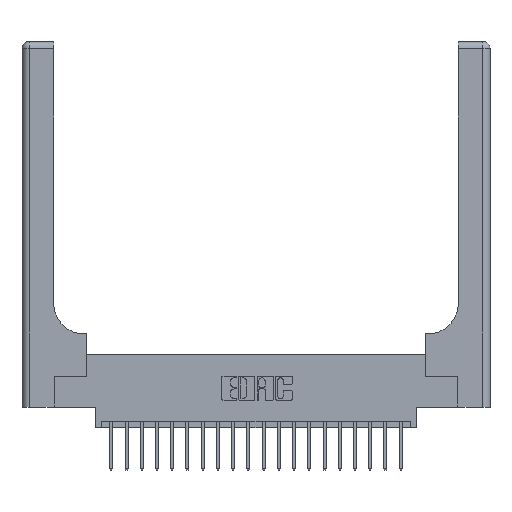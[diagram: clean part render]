
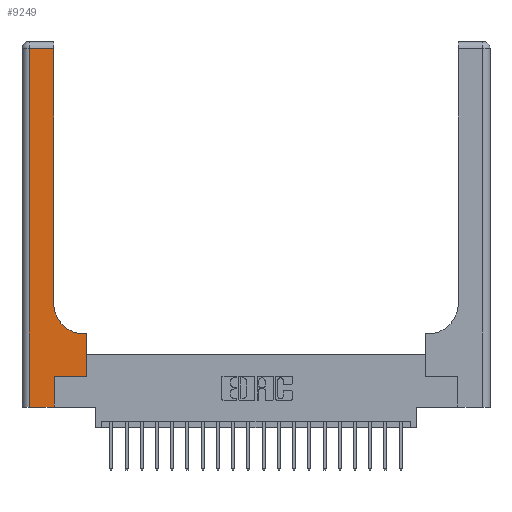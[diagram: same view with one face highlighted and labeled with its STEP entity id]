
A CAD part, top view. The second image highlights one B-rep face of the part: STEP entity #9249.
In plain terms, the highlighted planar face has unit normal (0, 0, 1).
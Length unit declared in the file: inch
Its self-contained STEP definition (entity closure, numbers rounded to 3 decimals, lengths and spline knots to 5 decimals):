
#969 = ORIENTED_EDGE ( 'NONE', *, *, #4519, .T. ) ;
#1064 = CARTESIAN_POINT ( 'NONE',  ( 0.51, 0.6, 0.37 ) ) ;
#1404 = PLANE ( 'NONE',  #8314 ) ;
#1443 = VECTOR ( 'NONE', #10503, 39.37008 ) ;
#1856 = ORIENTED_EDGE ( 'NONE', *, *, #5648, .T. ) ;
#2175 = CARTESIAN_POINT ( 'NONE',  ( 0.26, 3., 0.37 ) ) ;
#2435 = CARTESIAN_POINT ( 'NONE',  ( 0.26, 0.85, 0.37 ) ) ;
#2613 = CARTESIAN_POINT ( 'NONE',  ( 0.26, 0.6, 0.37 ) ) ;
#3101 = DIRECTION ( 'NONE',  ( 0., 0., -1. ) ) ;
#3227 = DIRECTION ( 'NONE',  ( 0., 0., -1. ) ) ;
#3654 = VERTEX_POINT ( 'NONE', #8436 ) ;
#4396 = LINE ( 'NONE', #18512, #11097 ) ;
#4419 = VERTEX_POINT ( 'NONE', #5235 ) ;
#4519 = EDGE_CURVE ( 'NONE', #6497, #8329, #18994, .T. ) ;
#4797 = VECTOR ( 'NONE', #16852, 39.37008 ) ;
#5235 = CARTESIAN_POINT ( 'NONE',  ( 0.265, 0., 0.37 ) ) ;
#5289 = VERTEX_POINT ( 'NONE', #1064 ) ;
#5648 = EDGE_CURVE ( 'NONE', #20893, #11310, #8142, .T. ) ;
#5678 = CARTESIAN_POINT ( 'NONE',  ( 0.265, 0.25, 0.37 ) ) ;
#5838 = CARTESIAN_POINT ( 'NONE',  ( 0.528, 0.25, 0.37 ) ) ;
#6059 = LINE ( 'NONE', #2613, #14283 ) ;
#6120 = CARTESIAN_POINT ( 'NONE',  ( 0.528, 0.6, 0.37 ) ) ;
#6497 = VERTEX_POINT ( 'NONE', #2435 ) ;
#6508 = EDGE_LOOP ( 'NONE', ( #969, #9099, #1856, #19226, #16027, #8920, #12571, #19442, #12322 ) ) ;
#6956 = CARTESIAN_POINT ( 'NONE',  ( 0.265, 0., 0.37 ) ) ;
#7095 = DIRECTION ( 'NONE',  ( 1., 0., 0. ) ) ;
#7485 = DIRECTION ( 'NONE',  ( 0., 1., 0. ) ) ;
#7694 = EDGE_CURVE ( 'NONE', #13878, #5289, #6059, .T. ) ;
#7697 = EDGE_CURVE ( 'NONE', #8329, #20893, #19194, .T. ) ;
#7995 = CIRCLE ( 'NONE', #12030, 0.25 ) ;
#8142 = LINE ( 'NONE', #15171, #4797 ) ;
#8241 = EDGE_CURVE ( 'NONE', #11310, #4419, #9414, .T. ) ;
#8314 = AXIS2_PLACEMENT_3D ( 'NONE', #16167, #3101, #14602 ) ;
#8329 = VERTEX_POINT ( 'NONE', #8822 ) ;
#8365 = VECTOR ( 'NONE', #7095, 39.37008 ) ;
#8436 = CARTESIAN_POINT ( 'NONE',  ( 0.528, 0.25, 0.37 ) ) ;
#8703 = CARTESIAN_POINT ( 'NONE',  ( 0.06, 0., 0.37 ) ) ;
#8822 = CARTESIAN_POINT ( 'NONE',  ( 0.26, 2.94, 0.37 ) ) ;
#8920 = ORIENTED_EDGE ( 'NONE', *, *, #10804, .T. ) ;
#9099 = ORIENTED_EDGE ( 'NONE', *, *, #7697, .T. ) ;
#9249 = ADVANCED_FACE ( 'NONE', ( #20881 ), #1404, .F. ) ;
#9271 = DIRECTION ( 'NONE',  ( -1., 0., 0. ) ) ;
#9414 = LINE ( 'NONE', #18601, #8365 ) ;
#9637 = VERTEX_POINT ( 'NONE', #5678 ) ;
#10503 = DIRECTION ( 'NONE',  ( 0., 1., 0. ) ) ;
#10804 = EDGE_CURVE ( 'NONE', #9637, #3654, #4396, .T. ) ;
#11097 = VECTOR ( 'NONE', #20132, 39.37008 ) ;
#11310 = VERTEX_POINT ( 'NONE', #8703 ) ;
#11463 = LINE ( 'NONE', #6956, #15261 ) ;
#11480 = VECTOR ( 'NONE', #9271, 39.37008 ) ;
#11729 = EDGE_CURVE ( 'NONE', #5289, #6497, #7995, .T. ) ;
#12030 = AXIS2_PLACEMENT_3D ( 'NONE', #13060, #3227, #14724 ) ;
#12201 = VECTOR ( 'NONE', #7485, 39.37008 ) ;
#12322 = ORIENTED_EDGE ( 'NONE', *, *, #11729, .T. ) ;
#12571 = ORIENTED_EDGE ( 'NONE', *, *, #19417, .T. ) ;
#13060 = CARTESIAN_POINT ( 'NONE',  ( 0.51, 0.85, 0.37 ) ) ;
#13878 = VERTEX_POINT ( 'NONE', #6120 ) ;
#14114 = CARTESIAN_POINT ( 'NONE',  ( 0., 2.94, 0.37 ) ) ;
#14283 = VECTOR ( 'NONE', #17371, 39.37008 ) ;
#14602 = DIRECTION ( 'NONE',  ( -1., 0., 0. ) ) ;
#14724 = DIRECTION ( 'NONE',  ( 1., 0., 0. ) ) ;
#15171 = CARTESIAN_POINT ( 'NONE',  ( 0.06, 3., 0.37 ) ) ;
#15261 = VECTOR ( 'NONE', #16790, 39.37008 ) ;
#16027 = ORIENTED_EDGE ( 'NONE', *, *, #18656, .T. ) ;
#16167 = CARTESIAN_POINT ( 'NONE',  ( 0., 3., 0.37 ) ) ;
#16790 = DIRECTION ( 'NONE',  ( 0., 1., 0. ) ) ;
#16852 = DIRECTION ( 'NONE',  ( 0., -1., 0. ) ) ;
#17371 = DIRECTION ( 'NONE',  ( -1., 0., 0. ) ) ;
#17875 = CARTESIAN_POINT ( 'NONE',  ( 0.06, 2.94, 0.37 ) ) ;
#18512 = CARTESIAN_POINT ( 'NONE',  ( 0.265, 0.25, 0.37 ) ) ;
#18601 = CARTESIAN_POINT ( 'NONE',  ( 0., 0., 0.37 ) ) ;
#18656 = EDGE_CURVE ( 'NONE', #4419, #9637, #11463, .T. ) ;
#18994 = LINE ( 'NONE', #2175, #1443 ) ;
#19194 = LINE ( 'NONE', #14114, #11480 ) ;
#19226 = ORIENTED_EDGE ( 'NONE', *, *, #8241, .T. ) ;
#19417 = EDGE_CURVE ( 'NONE', #3654, #13878, #20923, .T. ) ;
#19442 = ORIENTED_EDGE ( 'NONE', *, *, #7694, .T. ) ;
#20132 = DIRECTION ( 'NONE',  ( 1., 0., 0. ) ) ;
#20881 = FACE_OUTER_BOUND ( 'NONE', #6508, .T. ) ;
#20893 = VERTEX_POINT ( 'NONE', #17875 ) ;
#20923 = LINE ( 'NONE', #5838, #12201 ) ;
